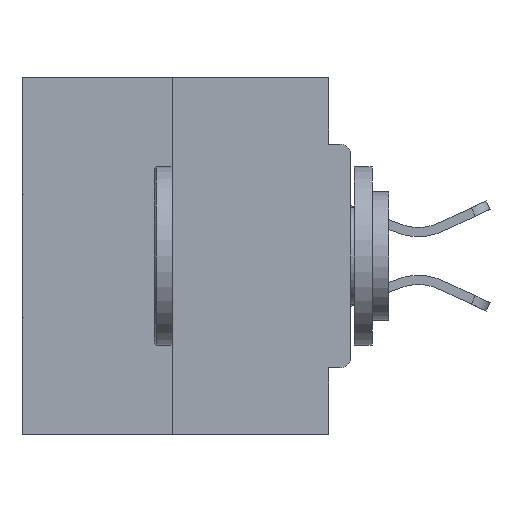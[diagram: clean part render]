
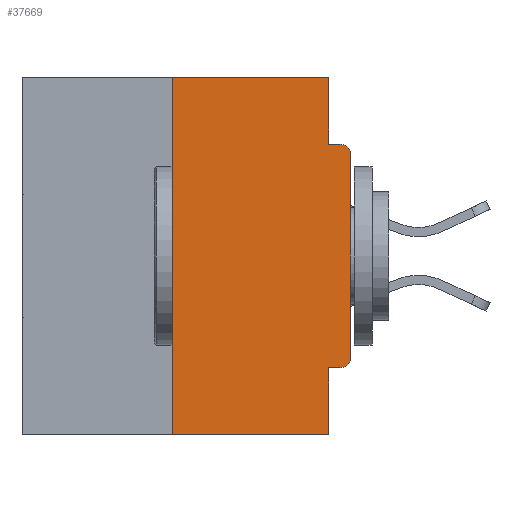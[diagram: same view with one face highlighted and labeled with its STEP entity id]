
A CAD part, left-side view. The second image highlights one B-rep face of the part: STEP entity #37669.
In plain terms, the highlighted planar face has unit normal (-1, 0, 0).
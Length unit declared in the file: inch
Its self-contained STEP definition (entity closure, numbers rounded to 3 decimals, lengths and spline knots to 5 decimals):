
#206 = CARTESIAN_POINT ( 'NONE',  ( 0., 0.031, -0.5 ) ) ;
#814 = VERTEX_POINT ( 'NONE', #14674 ) ;
#830 = ORIENTED_EDGE ( 'NONE', *, *, #22843, .F. ) ;
#1253 = ORIENTED_EDGE ( 'NONE', *, *, #15845, .F. ) ;
#1575 = CARTESIAN_POINT ( 'NONE',  ( 0., 0.015, -0.1085 ) ) ;
#1935 = CIRCLE ( 'NONE', #30055, 0.015 ) ;
#2377 = EDGE_LOOP ( 'NONE', ( #37539, #27105, #13398, #1253, #4279, #12875, #25596, #19460, #9223, #830 ) ) ;
#2697 = VECTOR ( 'NONE', #33467, 39.37008 ) ;
#3426 = DIRECTION ( 'NONE',  ( 0., 0., -1. ) ) ;
#4222 = CARTESIAN_POINT ( 'NONE',  ( 0., 0.031, -0.0935 ) ) ;
#4279 = ORIENTED_EDGE ( 'NONE', *, *, #8130, .F. ) ;
#5156 = CIRCLE ( 'NONE', #15952, 0.015 ) ;
#5760 = DIRECTION ( 'NONE',  ( 0., 0., 1. ) ) ;
#5834 = VECTOR ( 'NONE', #6349, 39.37008 ) ;
#6053 = VERTEX_POINT ( 'NONE', #18527 ) ;
#6213 = LINE ( 'NONE', #206, #32568 ) ;
#6349 = DIRECTION ( 'NONE',  ( 0., -1., 0. ) ) ;
#6820 = VECTOR ( 'NONE', #34938, 39.37008 ) ;
#7838 = CARTESIAN_POINT ( 'NONE',  ( 0., 0.015, -0.0935 ) ) ;
#8130 = EDGE_CURVE ( 'NONE', #11307, #35814, #25702, .T. ) ;
#8505 = PLANE ( 'NONE',  #36585 ) ;
#8767 = CARTESIAN_POINT ( 'NONE',  ( 0., 0.46, 0. ) ) ;
#8857 = CARTESIAN_POINT ( 'NONE',  ( 0., 0.015, -0.3915 ) ) ;
#9223 = ORIENTED_EDGE ( 'NONE', *, *, #34116, .F. ) ;
#9407 = CARTESIAN_POINT ( 'NONE',  ( 0., 0.25, 0. ) ) ;
#9514 = VECTOR ( 'NONE', #5760, 39.37008 ) ;
#11307 = VERTEX_POINT ( 'NONE', #25392 ) ;
#11573 = VECTOR ( 'NONE', #33133, 39.37008 ) ;
#11731 = LINE ( 'NONE', #24072, #37117 ) ;
#12326 = DIRECTION ( 'NONE',  ( 0., 0., 1. ) ) ;
#12615 = EDGE_CURVE ( 'NONE', #6053, #37712, #22528, .T. ) ;
#12875 = ORIENTED_EDGE ( 'NONE', *, *, #37216, .T. ) ;
#13398 = ORIENTED_EDGE ( 'NONE', *, *, #20020, .T. ) ;
#14429 = DIRECTION ( 'NONE',  ( 0., 0., -1. ) ) ;
#14674 = CARTESIAN_POINT ( 'NONE',  ( 0., 0.031, -0.5 ) ) ;
#14691 = LINE ( 'NONE', #17911, #9514 ) ;
#14695 = LINE ( 'NONE', #9407, #23650 ) ;
#15845 = EDGE_CURVE ( 'NONE', #35814, #814, #6213, .T. ) ;
#15952 = AXIS2_PLACEMENT_3D ( 'NONE', #8857, #20579, #32383 ) ;
#17911 = CARTESIAN_POINT ( 'NONE',  ( 0., 0., 0. ) ) ;
#18012 = DIRECTION ( 'NONE',  ( 0., -1., 0. ) ) ;
#18527 = CARTESIAN_POINT ( 'NONE',  ( 0., 0.25, 0. ) ) ;
#19460 = ORIENTED_EDGE ( 'NONE', *, *, #38898, .T. ) ;
#19998 = CARTESIAN_POINT ( 'NONE',  ( 0., 0., -0.1085 ) ) ;
#20020 = EDGE_CURVE ( 'NONE', #31497, #814, #11731, .T. ) ;
#20023 = CARTESIAN_POINT ( 'NONE',  ( 0., 0.25, -0.5 ) ) ;
#20579 = DIRECTION ( 'NONE',  ( -1., 0., 0. ) ) ;
#21175 = CARTESIAN_POINT ( 'NONE',  ( 0., 0., -0.4065 ) ) ;
#21514 = CARTESIAN_POINT ( 'NONE',  ( 0., 0.46, 0. ) ) ;
#22528 = LINE ( 'NONE', #21514, #2697 ) ;
#22566 = DIRECTION ( 'NONE',  ( -1., 0., 0. ) ) ;
#22843 = EDGE_CURVE ( 'NONE', #37712, #37829, #23298, .T. ) ;
#22858 = VERTEX_POINT ( 'NONE', #7838 ) ;
#23065 = FACE_OUTER_BOUND ( 'NONE', #2377, .T. ) ;
#23298 = LINE ( 'NONE', #34539, #6820 ) ;
#23394 = DIRECTION ( 'NONE',  ( 1., 0., 0. ) ) ;
#23650 = VECTOR ( 'NONE', #12326, 39.37008 ) ;
#24072 = CARTESIAN_POINT ( 'NONE',  ( 0., 0.46, -0.5 ) ) ;
#24528 = EDGE_CURVE ( 'NONE', #31497, #6053, #14695, .T. ) ;
#25392 = CARTESIAN_POINT ( 'NONE',  ( 0., 0.015, -0.4065 ) ) ;
#25596 = ORIENTED_EDGE ( 'NONE', *, *, #28673, .T. ) ;
#25606 = DIRECTION ( 'NONE',  ( 0., 0., -1. ) ) ;
#25702 = LINE ( 'NONE', #21175, #11573 ) ;
#26522 = CARTESIAN_POINT ( 'NONE',  ( 0., 0.031, 0. ) ) ;
#27027 = LINE ( 'NONE', #36738, #5834 ) ;
#27105 = ORIENTED_EDGE ( 'NONE', *, *, #24528, .F. ) ;
#28673 = EDGE_CURVE ( 'NONE', #35217, #38187, #14691, .T. ) ;
#30055 = AXIS2_PLACEMENT_3D ( 'NONE', #1575, #22566, #25606 ) ;
#31497 = VERTEX_POINT ( 'NONE', #20023 ) ;
#32383 = DIRECTION ( 'NONE',  ( 0., 0., -1. ) ) ;
#32568 = VECTOR ( 'NONE', #3426, 39.37008 ) ;
#33053 = CARTESIAN_POINT ( 'NONE',  ( 0., 0., -0.3915 ) ) ;
#33133 = DIRECTION ( 'NONE',  ( 0., 1., 0. ) ) ;
#33467 = DIRECTION ( 'NONE',  ( 0., -1., 0. ) ) ;
#34116 = EDGE_CURVE ( 'NONE', #37829, #22858, #27027, .T. ) ;
#34539 = CARTESIAN_POINT ( 'NONE',  ( 0., 0.031, 0. ) ) ;
#34938 = DIRECTION ( 'NONE',  ( 0., 0., -1. ) ) ;
#35217 = VERTEX_POINT ( 'NONE', #33053 ) ;
#35393 = CARTESIAN_POINT ( 'NONE',  ( 0., 0.031, -0.4065 ) ) ;
#35814 = VERTEX_POINT ( 'NONE', #35393 ) ;
#36585 = AXIS2_PLACEMENT_3D ( 'NONE', #8767, #23394, #14429 ) ;
#36738 = CARTESIAN_POINT ( 'NONE',  ( 0., 0., -0.0935 ) ) ;
#37117 = VECTOR ( 'NONE', #18012, 39.37008 ) ;
#37216 = EDGE_CURVE ( 'NONE', #11307, #35217, #5156, .T. ) ;
#37539 = ORIENTED_EDGE ( 'NONE', *, *, #12615, .F. ) ;
#37669 = ADVANCED_FACE ( 'NONE', ( #23065 ), #8505, .F. ) ;
#37712 = VERTEX_POINT ( 'NONE', #26522 ) ;
#37829 = VERTEX_POINT ( 'NONE', #4222 ) ;
#38187 = VERTEX_POINT ( 'NONE', #19998 ) ;
#38898 = EDGE_CURVE ( 'NONE', #38187, #22858, #1935, .T. ) ;
